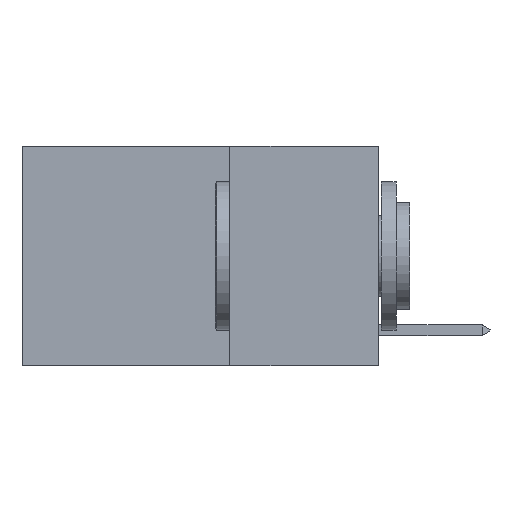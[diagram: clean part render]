
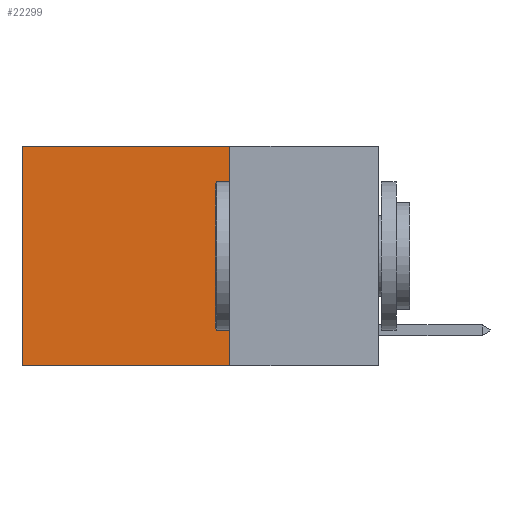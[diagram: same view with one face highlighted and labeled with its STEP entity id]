
A CAD part, left-side view. The second image highlights one B-rep face of the part: STEP entity #22299.
In plain terms, the highlighted planar face has unit normal (-1, 0, 0).
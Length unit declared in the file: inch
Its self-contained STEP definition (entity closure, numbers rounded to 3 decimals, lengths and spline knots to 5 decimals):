
#385 = DIRECTION ( 'NONE',  ( 0., 0., -1. ) ) ;
#1096 = CARTESIAN_POINT ( 'NONE',  ( 0.2625, 0.25, -0.37 ) ) ;
#1316 = EDGE_CURVE ( 'NONE', #24407, #22019, #10090, .T. ) ;
#2385 = DIRECTION ( 'NONE',  ( 0., 0., -1. ) ) ;
#2419 = CARTESIAN_POINT ( 'NONE',  ( 0.2625, 0.25, 0. ) ) ;
#3388 = VECTOR ( 'NONE', #22001, 39.37008 ) ;
#4493 = EDGE_CURVE ( 'NONE', #18300, #22019, #17167, .T. ) ;
#6608 = EDGE_CURVE ( 'NONE', #25404, #18300, #25240, .T. ) ;
#7291 = CARTESIAN_POINT ( 'NONE',  ( 0.2625, 0.25, 0. ) ) ;
#8368 = ORIENTED_EDGE ( 'NONE', *, *, #1316, .T. ) ;
#8640 = CARTESIAN_POINT ( 'NONE',  ( 0.2625, 0.6, -0.37 ) ) ;
#9604 = CARTESIAN_POINT ( 'NONE',  ( 0.2625, 0.6, 0. ) ) ;
#9638 = CARTESIAN_POINT ( 'NONE',  ( 0.2625, 0.6, 0. ) ) ;
#10090 = LINE ( 'NONE', #9638, #18637 ) ;
#10732 = LINE ( 'NONE', #24722, #3388 ) ;
#10864 = ORIENTED_EDGE ( 'NONE', *, *, #4493, .F. ) ;
#17167 = LINE ( 'NONE', #23923, #17876 ) ;
#17264 = AXIS2_PLACEMENT_3D ( 'NONE', #7291, #25930, #385 ) ;
#17353 = VECTOR ( 'NONE', #2385, 39.37008 ) ;
#17433 = DIRECTION ( 'NONE',  ( 0., 0., -1. ) ) ;
#17876 = VECTOR ( 'NONE', #27987, 39.37008 ) ;
#18016 = CARTESIAN_POINT ( 'NONE',  ( 0.2625, 0.25, 0. ) ) ;
#18300 = VERTEX_POINT ( 'NONE', #1096 ) ;
#18637 = VECTOR ( 'NONE', #17433, 39.37008 ) ;
#19929 = EDGE_LOOP ( 'NONE', ( #8368, #10864, #29432, #24512 ) ) ;
#22001 = DIRECTION ( 'NONE',  ( 0., 1., 0. ) ) ;
#22019 = VERTEX_POINT ( 'NONE', #8640 ) ;
#22299 = ADVANCED_FACE ( 'NONE', ( #23813 ), #23961, .F. ) ;
#23661 = EDGE_CURVE ( 'NONE', #25404, #24407, #10732, .T. ) ;
#23813 = FACE_OUTER_BOUND ( 'NONE', #19929, .T. ) ;
#23923 = CARTESIAN_POINT ( 'NONE',  ( 0.2625, 0.25, -0.37 ) ) ;
#23961 = PLANE ( 'NONE',  #17264 ) ;
#24407 = VERTEX_POINT ( 'NONE', #9604 ) ;
#24512 = ORIENTED_EDGE ( 'NONE', *, *, #23661, .T. ) ;
#24722 = CARTESIAN_POINT ( 'NONE',  ( 0.2625, 0.25, 0. ) ) ;
#25240 = LINE ( 'NONE', #18016, #17353 ) ;
#25404 = VERTEX_POINT ( 'NONE', #2419 ) ;
#25930 = DIRECTION ( 'NONE',  ( 1., 0., 0. ) ) ;
#27987 = DIRECTION ( 'NONE',  ( 0., 1., 0. ) ) ;
#29432 = ORIENTED_EDGE ( 'NONE', *, *, #6608, .F. ) ;
